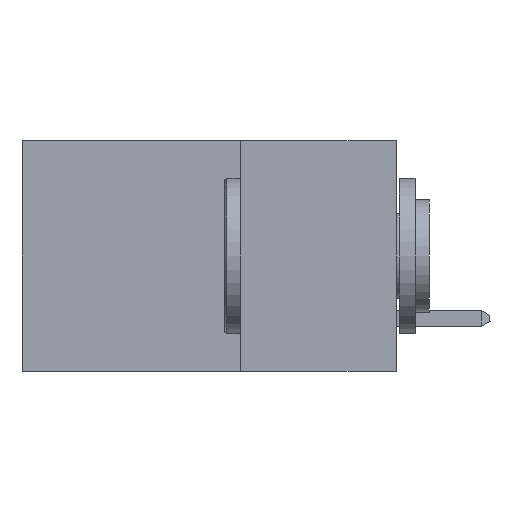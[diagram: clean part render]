
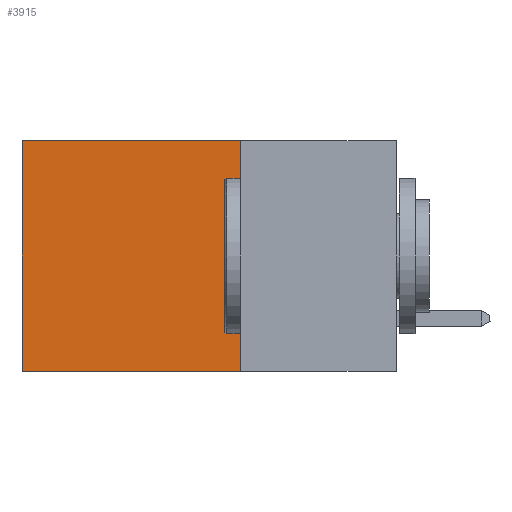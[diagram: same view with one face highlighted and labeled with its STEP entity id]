
A CAD part, left-side view. The second image highlights one B-rep face of the part: STEP entity #3915.
In plain terms, the highlighted planar face has unit normal (-1, 0, 0).
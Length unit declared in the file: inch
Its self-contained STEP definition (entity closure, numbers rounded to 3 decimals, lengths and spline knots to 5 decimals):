
#900 = VECTOR ( 'NONE', #7880, 39.37008 ) ;
#1042 = CARTESIAN_POINT ( 'NONE',  ( 0.298, 0.6, -0.37 ) ) ;
#1432 = VERTEX_POINT ( 'NONE', #3105 ) ;
#2040 = CARTESIAN_POINT ( 'NONE',  ( 0.298, 0.25, -0.37 ) ) ;
#2870 = ORIENTED_EDGE ( 'NONE', *, *, #10480, .F. ) ;
#2885 = FACE_OUTER_BOUND ( 'NONE', #10850, .T. ) ;
#3105 = CARTESIAN_POINT ( 'NONE',  ( 0.298, 0.6, 0. ) ) ;
#3431 = VERTEX_POINT ( 'NONE', #1042 ) ;
#3456 = LINE ( 'NONE', #7727, #8970 ) ;
#3915 = ADVANCED_FACE ( 'NONE', ( #2885 ), #11504, .F. ) ;
#4357 = VECTOR ( 'NONE', #8352, 39.37008 ) ;
#4595 = DIRECTION ( 'NONE',  ( 0., 1., 0. ) ) ;
#4655 = CARTESIAN_POINT ( 'NONE',  ( 0.298, 0.25, 0. ) ) ;
#4658 = VECTOR ( 'NONE', #5070, 39.37008 ) ;
#4731 = LINE ( 'NONE', #4655, #4357 ) ;
#5070 = DIRECTION ( 'NONE',  ( 0., 1., 0. ) ) ;
#5552 = DIRECTION ( 'NONE',  ( 1., 0., 0. ) ) ;
#5991 = VERTEX_POINT ( 'NONE', #2040 ) ;
#6232 = VERTEX_POINT ( 'NONE', #13082 ) ;
#6964 = LINE ( 'NONE', #11520, #900 ) ;
#7706 = ORIENTED_EDGE ( 'NONE', *, *, #8428, .F. ) ;
#7727 = CARTESIAN_POINT ( 'NONE',  ( 0.298, 0.25, 0. ) ) ;
#7754 = DIRECTION ( 'NONE',  ( 0., 0., -1. ) ) ;
#7880 = DIRECTION ( 'NONE',  ( 0., 0., -1. ) ) ;
#8352 = DIRECTION ( 'NONE',  ( 0., 0., -1. ) ) ;
#8428 = EDGE_CURVE ( 'NONE', #6232, #5991, #4731, .T. ) ;
#8970 = VECTOR ( 'NONE', #4595, 39.37008 ) ;
#9936 = CARTESIAN_POINT ( 'NONE',  ( 0.298, 0.25, -0.37 ) ) ;
#10480 = EDGE_CURVE ( 'NONE', #5991, #3431, #14434, .T. ) ;
#10850 = EDGE_LOOP ( 'NONE', ( #14407, #2870, #7706, #12259 ) ) ;
#11504 = PLANE ( 'NONE',  #11515 ) ;
#11515 = AXIS2_PLACEMENT_3D ( 'NONE', #12603, #5552, #7754 ) ;
#11520 = CARTESIAN_POINT ( 'NONE',  ( 0.298, 0.6, 0. ) ) ;
#12259 = ORIENTED_EDGE ( 'NONE', *, *, #15227, .T. ) ;
#12603 = CARTESIAN_POINT ( 'NONE',  ( 0.298, 0.25, 0. ) ) ;
#13082 = CARTESIAN_POINT ( 'NONE',  ( 0.298, 0.25, 0. ) ) ;
#13400 = EDGE_CURVE ( 'NONE', #1432, #3431, #6964, .T. ) ;
#14407 = ORIENTED_EDGE ( 'NONE', *, *, #13400, .T. ) ;
#14434 = LINE ( 'NONE', #9936, #4658 ) ;
#15227 = EDGE_CURVE ( 'NONE', #6232, #1432, #3456, .T. ) ;
